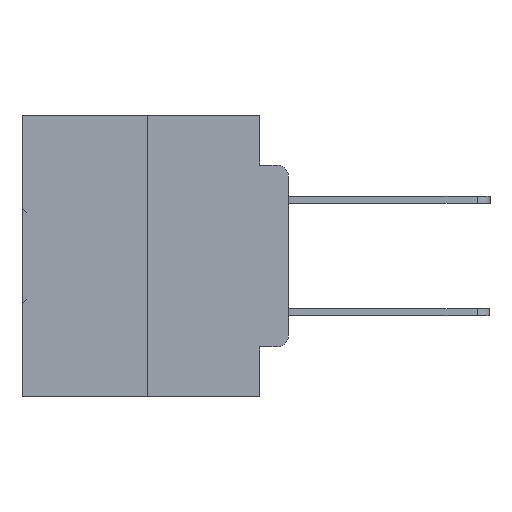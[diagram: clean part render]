
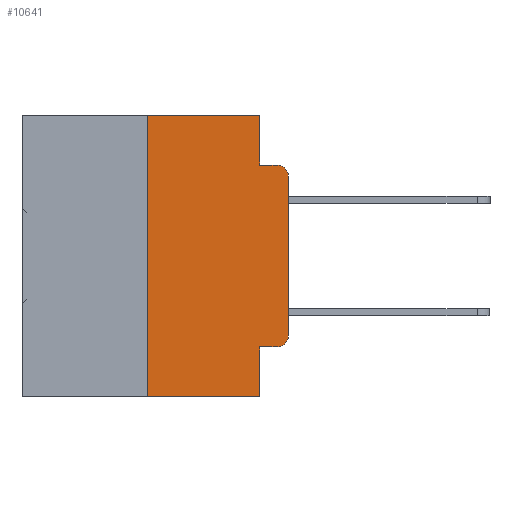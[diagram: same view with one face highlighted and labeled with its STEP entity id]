
A CAD part, left-side view. The second image highlights one B-rep face of the part: STEP entity #10641.
In plain terms, the highlighted planar face has unit normal (-1, 0, 0).
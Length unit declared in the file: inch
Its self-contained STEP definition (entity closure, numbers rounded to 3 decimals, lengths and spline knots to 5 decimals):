
#16 = EDGE_CURVE ( 'NONE', #16018, #32677, #4133, .T. ) ;
#246 = CARTESIAN_POINT ( 'NONE',  ( 0., 0.051, -0.4115 ) ) ;
#707 = AXIS2_PLACEMENT_3D ( 'NONE', #15473, #7620, #25980 ) ;
#834 = DIRECTION ( 'NONE',  ( 0., 0., -1. ) ) ;
#877 = DIRECTION ( 'NONE',  ( -1., 0., 0. ) ) ;
#947 = EDGE_CURVE ( 'NONE', #29603, #25668, #25990, .T. ) ;
#1407 = DIRECTION ( 'NONE',  ( 0., -1., 0. ) ) ;
#2546 = EDGE_CURVE ( 'NONE', #10301, #14861, #5832, .T. ) ;
#2746 = ORIENTED_EDGE ( 'NONE', *, *, #12281, .T. ) ;
#2751 = CARTESIAN_POINT ( 'NONE',  ( 0., 0.051, 0. ) ) ;
#2955 = VERTEX_POINT ( 'NONE', #25201 ) ;
#3396 = ORIENTED_EDGE ( 'NONE', *, *, #26529, .F. ) ;
#3487 = VECTOR ( 'NONE', #16151, 39.37008 ) ;
#3683 = CARTESIAN_POINT ( 'NONE',  ( 0., 0.25, -0.5 ) ) ;
#4133 = LINE ( 'NONE', #12732, #31399 ) ;
#4287 = VERTEX_POINT ( 'NONE', #246 ) ;
#4466 = ORIENTED_EDGE ( 'NONE', *, *, #2546, .T. ) ;
#4699 = ORIENTED_EDGE ( 'NONE', *, *, #16, .F. ) ;
#4866 = PLANE ( 'NONE',  #707 ) ;
#5060 = VERTEX_POINT ( 'NONE', #26875 ) ;
#5610 = LINE ( 'NONE', #22761, #17982 ) ;
#5832 = CIRCLE ( 'NONE', #25705, 0.02 ) ;
#6433 = ORIENTED_EDGE ( 'NONE', *, *, #9250, .T. ) ;
#6503 = CARTESIAN_POINT ( 'NONE',  ( 0., 0.051, -0.0885 ) ) ;
#7620 = DIRECTION ( 'NONE',  ( 1., 0., 0. ) ) ;
#7737 = CARTESIAN_POINT ( 'NONE',  ( 0., 0.02, -0.3915 ) ) ;
#8215 = CARTESIAN_POINT ( 'NONE',  ( 0., 0.02, -0.1085 ) ) ;
#9210 = DIRECTION ( 'NONE',  ( 0., -1., 0. ) ) ;
#9250 = EDGE_CURVE ( 'NONE', #16018, #5060, #12098, .T. ) ;
#9385 = ORIENTED_EDGE ( 'NONE', *, *, #21479, .F. ) ;
#9895 = CARTESIAN_POINT ( 'NONE',  ( 0., 0.473, -0.5 ) ) ;
#10301 = VERTEX_POINT ( 'NONE', #27211 ) ;
#10428 = DIRECTION ( 'NONE',  ( 0., 0., -1. ) ) ;
#10468 = VECTOR ( 'NONE', #30843, 39.37008 ) ;
#10641 = ADVANCED_FACE ( 'NONE', ( #22625 ), #4866, .F. ) ;
#11504 = LINE ( 'NONE', #29167, #3487 ) ;
#12098 = LINE ( 'NONE', #9895, #10468 ) ;
#12250 = ORIENTED_EDGE ( 'NONE', *, *, #947, .F. ) ;
#12281 = EDGE_CURVE ( 'NONE', #2955, #10301, #22567, .T. ) ;
#12732 = CARTESIAN_POINT ( 'NONE',  ( 0., 0.25, 0. ) ) ;
#12848 = DIRECTION ( 'NONE',  ( 0., 0., -1. ) ) ;
#12851 = LINE ( 'NONE', #6503, #25934 ) ;
#13229 = DIRECTION ( 'NONE',  ( 0., 0., -1. ) ) ;
#13758 = DIRECTION ( 'NONE',  ( 0., 0., 1. ) ) ;
#13867 = LINE ( 'NONE', #14829, #25312 ) ;
#14502 = EDGE_CURVE ( 'NONE', #34110, #2955, #19656, .T. ) ;
#14597 = CARTESIAN_POINT ( 'NONE',  ( 0., 0.25, 0. ) ) ;
#14829 = CARTESIAN_POINT ( 'NONE',  ( 0., 0.051, -0.4115 ) ) ;
#14861 = VERTEX_POINT ( 'NONE', #30544 ) ;
#15473 = CARTESIAN_POINT ( 'NONE',  ( 0., 0.473, 0. ) ) ;
#15595 = CARTESIAN_POINT ( 'NONE',  ( 0., 0.02, -0.4115 ) ) ;
#15638 = CARTESIAN_POINT ( 'NONE',  ( 0., 0.051, 0. ) ) ;
#15696 = EDGE_LOOP ( 'NONE', ( #2746, #4466, #3396, #12250, #9385, #4699, #6433, #27413, #30710, #19201 ) ) ;
#16018 = VERTEX_POINT ( 'NONE', #3683 ) ;
#16151 = DIRECTION ( 'NONE',  ( 0., -1., 0. ) ) ;
#17982 = VECTOR ( 'NONE', #12848, 39.37008 ) ;
#19201 = ORIENTED_EDGE ( 'NONE', *, *, #14502, .T. ) ;
#19656 = CIRCLE ( 'NONE', #21778, 0.02 ) ;
#21479 = EDGE_CURVE ( 'NONE', #32677, #29603, #11504, .T. ) ;
#21778 = AXIS2_PLACEMENT_3D ( 'NONE', #7737, #26082, #10428 ) ;
#22119 = EDGE_CURVE ( 'NONE', #4287, #5060, #5610, .T. ) ;
#22438 = CARTESIAN_POINT ( 'NONE',  ( 0., 0., 0. ) ) ;
#22567 = LINE ( 'NONE', #22438, #26255 ) ;
#22625 = FACE_OUTER_BOUND ( 'NONE', #15696, .T. ) ;
#22761 = CARTESIAN_POINT ( 'NONE',  ( 0., 0.051, 0. ) ) ;
#23250 = EDGE_CURVE ( 'NONE', #4287, #34110, #13867, .T. ) ;
#23339 = CARTESIAN_POINT ( 'NONE',  ( 0., 0.051, -0.0885 ) ) ;
#25201 = CARTESIAN_POINT ( 'NONE',  ( 0., 0., -0.3915 ) ) ;
#25312 = VECTOR ( 'NONE', #1407, 39.37008 ) ;
#25668 = VERTEX_POINT ( 'NONE', #23339 ) ;
#25705 = AXIS2_PLACEMENT_3D ( 'NONE', #8215, #877, #834 ) ;
#25934 = VECTOR ( 'NONE', #9210, 39.37008 ) ;
#25980 = DIRECTION ( 'NONE',  ( 0., 0., -1. ) ) ;
#25990 = LINE ( 'NONE', #15638, #32921 ) ;
#26082 = DIRECTION ( 'NONE',  ( -1., 0., 0. ) ) ;
#26255 = VECTOR ( 'NONE', #30350, 39.37008 ) ;
#26529 = EDGE_CURVE ( 'NONE', #25668, #14861, #12851, .T. ) ;
#26875 = CARTESIAN_POINT ( 'NONE',  ( 0., 0.051, -0.5 ) ) ;
#27211 = CARTESIAN_POINT ( 'NONE',  ( 0., 0., -0.1085 ) ) ;
#27413 = ORIENTED_EDGE ( 'NONE', *, *, #22119, .F. ) ;
#29167 = CARTESIAN_POINT ( 'NONE',  ( 0., 0.473, 0. ) ) ;
#29603 = VERTEX_POINT ( 'NONE', #2751 ) ;
#30350 = DIRECTION ( 'NONE',  ( 0., 0., 1. ) ) ;
#30544 = CARTESIAN_POINT ( 'NONE',  ( 0., 0.02, -0.0885 ) ) ;
#30710 = ORIENTED_EDGE ( 'NONE', *, *, #23250, .T. ) ;
#30843 = DIRECTION ( 'NONE',  ( 0., -1., 0. ) ) ;
#31399 = VECTOR ( 'NONE', #13758, 39.37008 ) ;
#32677 = VERTEX_POINT ( 'NONE', #14597 ) ;
#32921 = VECTOR ( 'NONE', #13229, 39.37008 ) ;
#34110 = VERTEX_POINT ( 'NONE', #15595 ) ;
